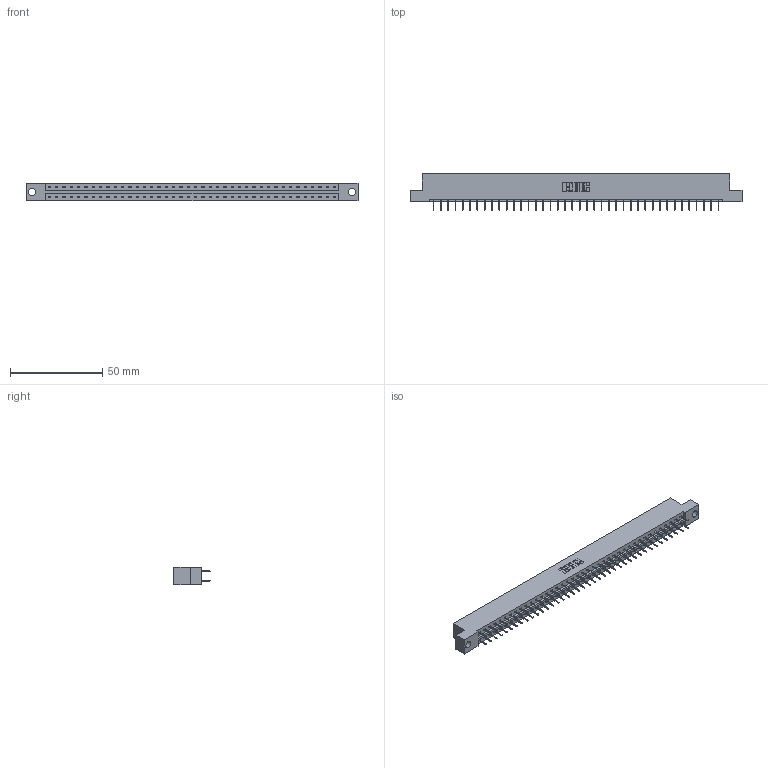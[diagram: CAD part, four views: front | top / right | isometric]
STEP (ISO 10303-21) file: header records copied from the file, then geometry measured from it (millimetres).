
FILE_DESCRIPTION (( 'STEP AP203' ), '1' );
FILE_NAME ('333-080-524-204.STEP', '2018-08-05T01:27:59', ( '' ), ( '' ), 'SwSTEP 2.0', 'SolidWorks 2016', '' );
FILE_SCHEMA (( 'CONFIG_CONTROL_DESIGN' ));
Length unit declared in the file: inch
Products named in the file (3): 333 Part_Flush - .156 Dia - TH; 345-292-001_345-293-124; 333-080-524-204
Assembly tree (81 placements, depth 2):
  333-080-524-204
    333 Part_Flush - .156 Dia - TH
    345-292-001_345-293-124  x80
Bounding box: 180.04 x 19.69 x 9.4 mm (x, y, z)
Volume: 18152.9 mm3; surface area: 20875.9 mm2
Topology: 81 solids, 81 shells, 4594 faces, 13031 edges, 8366 vertices
Faces by surface type: plane 3430, cylinder 1164
Entity records: 26069 total; most frequent: CARTESIAN_POINT 4322, ORIENTED_EDGE 4258, DIRECTION 3697, EDGE_CURVE 2129, LINE 2005, VECTOR 2005, VERTEX_POINT 1414, AXIS2_PLACEMENT_3D 846
